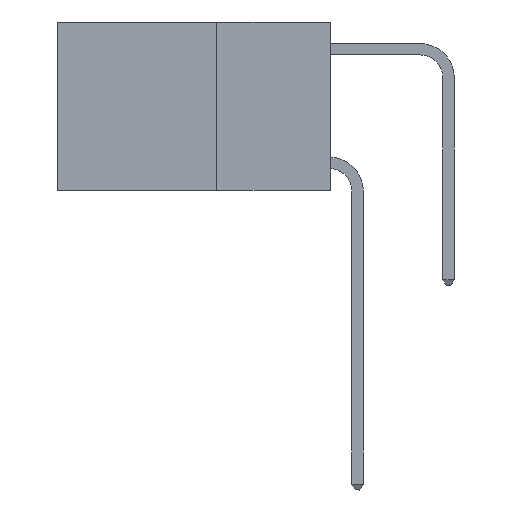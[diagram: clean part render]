
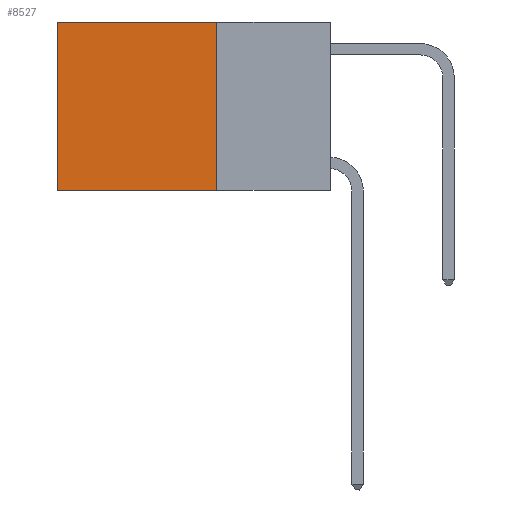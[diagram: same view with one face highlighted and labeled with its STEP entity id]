
A CAD part, left-side view. The second image highlights one B-rep face of the part: STEP entity #8527.
In plain terms, the highlighted planar face has unit normal (-1, 0, 0).
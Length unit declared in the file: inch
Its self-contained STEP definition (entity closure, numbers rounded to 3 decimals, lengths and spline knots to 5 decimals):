
#212 = EDGE_LOOP ( 'NONE', ( #5649, #5825, #6740, #6932 ) ) ;
#306 = PLANE ( 'NONE',  #7419 ) ;
#612 = LINE ( 'NONE', #7697, #6449 ) ;
#1320 = VECTOR ( 'NONE', #2802, 39.37008 ) ;
#2075 = CARTESIAN_POINT ( 'NONE',  ( 0.2625, 0.6, 0. ) ) ;
#2151 = VERTEX_POINT ( 'NONE', #3923 ) ;
#2559 = EDGE_CURVE ( 'NONE', #7192, #2151, #12634, .T. ) ;
#2772 = DIRECTION ( 'NONE',  ( 1., 0., 0. ) ) ;
#2802 = DIRECTION ( 'NONE',  ( 0., 1., 0. ) ) ;
#3896 = FACE_OUTER_BOUND ( 'NONE', #212, .T. ) ;
#3923 = CARTESIAN_POINT ( 'NONE',  ( 0.2625, 0.6, 0. ) ) ;
#4903 = DIRECTION ( 'NONE',  ( 0., 1., 0. ) ) ;
#5242 = CARTESIAN_POINT ( 'NONE',  ( 0.2625, 0.25, 0. ) ) ;
#5649 = ORIENTED_EDGE ( 'NONE', *, *, #12523, .T. ) ;
#5709 = CARTESIAN_POINT ( 'NONE',  ( 0.2625, 0.6, -0.37 ) ) ;
#5825 = ORIENTED_EDGE ( 'NONE', *, *, #7098, .F. ) ;
#6449 = VECTOR ( 'NONE', #10987, 39.37008 ) ;
#6740 = ORIENTED_EDGE ( 'NONE', *, *, #11107, .F. ) ;
#6932 = ORIENTED_EDGE ( 'NONE', *, *, #2559, .T. ) ;
#7098 = EDGE_CURVE ( 'NONE', #11592, #11933, #12885, .T. ) ;
#7192 = VERTEX_POINT ( 'NONE', #5242 ) ;
#7357 = CARTESIAN_POINT ( 'NONE',  ( 0.2625, 0.25, -0.37 ) ) ;
#7419 = AXIS2_PLACEMENT_3D ( 'NONE', #8329, #2772, #10531 ) ;
#7697 = CARTESIAN_POINT ( 'NONE',  ( 0.2625, 0.25, 0. ) ) ;
#7973 = VECTOR ( 'NONE', #12101, 39.37008 ) ;
#8164 = CARTESIAN_POINT ( 'NONE',  ( 0.2625, 0.25, 0. ) ) ;
#8329 = CARTESIAN_POINT ( 'NONE',  ( 0.2625, 0.25, 0. ) ) ;
#8527 = ADVANCED_FACE ( 'NONE', ( #3896 ), #306, .F. ) ;
#10531 = DIRECTION ( 'NONE',  ( 0., 0., -1. ) ) ;
#10566 = CARTESIAN_POINT ( 'NONE',  ( 0.2625, 0.25, -0.37 ) ) ;
#10875 = LINE ( 'NONE', #2075, #7973 ) ;
#10987 = DIRECTION ( 'NONE',  ( 0., 0., -1. ) ) ;
#11107 = EDGE_CURVE ( 'NONE', #7192, #11592, #612, .T. ) ;
#11592 = VERTEX_POINT ( 'NONE', #7357 ) ;
#11933 = VERTEX_POINT ( 'NONE', #5709 ) ;
#12101 = DIRECTION ( 'NONE',  ( 0., 0., -1. ) ) ;
#12283 = VECTOR ( 'NONE', #4903, 39.37008 ) ;
#12523 = EDGE_CURVE ( 'NONE', #2151, #11933, #10875, .T. ) ;
#12634 = LINE ( 'NONE', #8164, #12283 ) ;
#12885 = LINE ( 'NONE', #10566, #1320 ) ;
